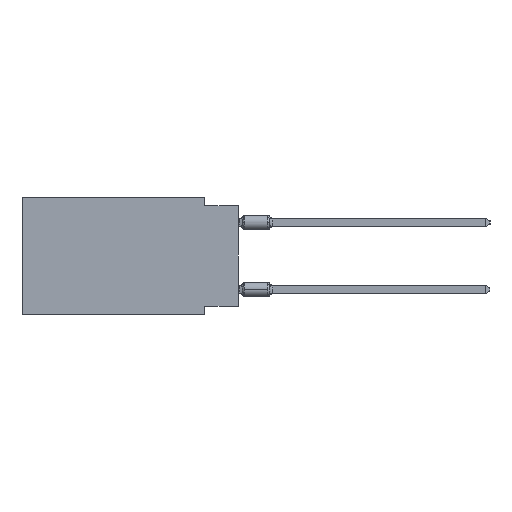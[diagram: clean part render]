
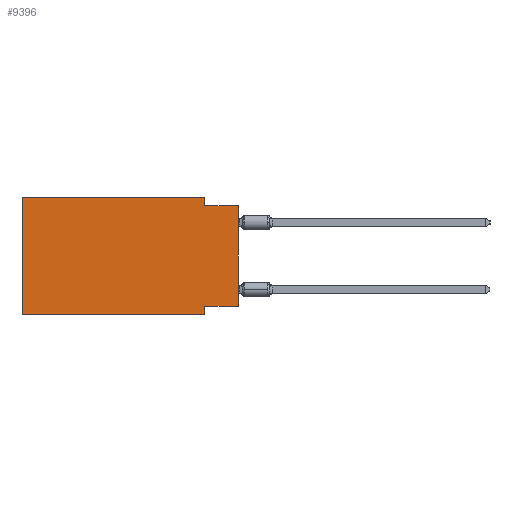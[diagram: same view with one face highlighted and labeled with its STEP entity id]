
A CAD part, left-side view. The second image highlights one B-rep face of the part: STEP entity #9396.
In plain terms, the highlighted planar face has unit normal (-1, 0, 0).
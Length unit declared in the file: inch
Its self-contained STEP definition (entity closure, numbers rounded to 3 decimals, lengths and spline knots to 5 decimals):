
#446 = CARTESIAN_POINT ( 'NONE',  ( 0., 0., -0.325 ) ) ;
#1252 = ORIENTED_EDGE ( 'NONE', *, *, #28286, .F. ) ;
#1313 = VECTOR ( 'NONE', #11956, 39.37008 ) ;
#2677 = CARTESIAN_POINT ( 'NONE',  ( 0., 0.1, -0.35 ) ) ;
#3009 = VERTEX_POINT ( 'NONE', #25775 ) ;
#3066 = DIRECTION ( 'NONE',  ( 0., 1., 0. ) ) ;
#3431 = DIRECTION ( 'NONE',  ( 0., -1., 0. ) ) ;
#3867 = EDGE_CURVE ( 'NONE', #3009, #34029, #23481, .T. ) ;
#5964 = AXIS2_PLACEMENT_3D ( 'NONE', #33407, #11883, #37676 ) ;
#6790 = VECTOR ( 'NONE', #33878, 39.37008 ) ;
#7600 = VERTEX_POINT ( 'NONE', #25044 ) ;
#8003 = VECTOR ( 'NONE', #27039, 39.37008 ) ;
#8285 = VERTEX_POINT ( 'NONE', #33639 ) ;
#9396 = ADVANCED_FACE ( 'NONE', ( #19673 ), #16127, .F. ) ;
#10119 = DIRECTION ( 'NONE',  ( 0., -1., 0. ) ) ;
#10926 = VERTEX_POINT ( 'NONE', #19369 ) ;
#11883 = DIRECTION ( 'NONE',  ( 1., 0., 0. ) ) ;
#11956 = DIRECTION ( 'NONE',  ( 0., 0., -1. ) ) ;
#13895 = CARTESIAN_POINT ( 'NONE',  ( 0., 0.645, -0.35 ) ) ;
#15711 = CARTESIAN_POINT ( 'NONE',  ( 0., 0.645, -0.35 ) ) ;
#16127 = PLANE ( 'NONE',  #5964 ) ;
#17143 = EDGE_CURVE ( 'NONE', #43151, #31957, #22496, .T. ) ;
#17479 = ORIENTED_EDGE ( 'NONE', *, *, #22959, .F. ) ;
#17889 = CARTESIAN_POINT ( 'NONE',  ( 0., 0.1, -0.025 ) ) ;
#18559 = CARTESIAN_POINT ( 'NONE',  ( 0., 0.645, 0. ) ) ;
#19369 = CARTESIAN_POINT ( 'NONE',  ( 0., 0.1, 0. ) ) ;
#19673 = FACE_OUTER_BOUND ( 'NONE', #28832, .T. ) ;
#20497 = VECTOR ( 'NONE', #3066, 39.37008 ) ;
#21859 = VECTOR ( 'NONE', #3431, 39.37008 ) ;
#21965 = LINE ( 'NONE', #446, #20497 ) ;
#22496 = LINE ( 'NONE', #37662, #6790 ) ;
#22507 = EDGE_CURVE ( 'NONE', #44842, #7600, #29139, .T. ) ;
#22959 = EDGE_CURVE ( 'NONE', #8285, #3009, #21965, .T. ) ;
#23430 = EDGE_CURVE ( 'NONE', #43151, #34029, #31881, .T. ) ;
#23481 = LINE ( 'NONE', #2677, #8003 ) ;
#24514 = LINE ( 'NONE', #42287, #38938 ) ;
#25044 = CARTESIAN_POINT ( 'NONE',  ( 0., 0., -0.025 ) ) ;
#25245 = ORIENTED_EDGE ( 'NONE', *, *, #17143, .F. ) ;
#25775 = CARTESIAN_POINT ( 'NONE',  ( 0., 0.1, -0.325 ) ) ;
#25798 = VECTOR ( 'NONE', #10119, 39.37008 ) ;
#27039 = DIRECTION ( 'NONE',  ( 0., 0., -1. ) ) ;
#27448 = ORIENTED_EDGE ( 'NONE', *, *, #37164, .F. ) ;
#27828 = ORIENTED_EDGE ( 'NONE', *, *, #23430, .T. ) ;
#28286 = EDGE_CURVE ( 'NONE', #10926, #44842, #40580, .T. ) ;
#28309 = ORIENTED_EDGE ( 'NONE', *, *, #43492, .T. ) ;
#28832 = EDGE_LOOP ( 'NONE', ( #28309, #33011, #1252, #27448, #25245, #27828, #40102, #17479 ) ) ;
#29139 = LINE ( 'NONE', #42876, #38626 ) ;
#29693 = CARTESIAN_POINT ( 'NONE',  ( 0., 0.1, 0. ) ) ;
#31881 = LINE ( 'NONE', #13895, #25798 ) ;
#31957 = VERTEX_POINT ( 'NONE', #44024 ) ;
#33011 = ORIENTED_EDGE ( 'NONE', *, *, #22507, .F. ) ;
#33178 = CARTESIAN_POINT ( 'NONE',  ( 0., 0.1, -0.35 ) ) ;
#33407 = CARTESIAN_POINT ( 'NONE',  ( 0., 0.645, 0. ) ) ;
#33639 = CARTESIAN_POINT ( 'NONE',  ( 0., 0., -0.325 ) ) ;
#33878 = DIRECTION ( 'NONE',  ( 0., 0., 1. ) ) ;
#34029 = VERTEX_POINT ( 'NONE', #33178 ) ;
#36321 = LINE ( 'NONE', #18559, #21859 ) ;
#37164 = EDGE_CURVE ( 'NONE', #31957, #10926, #36321, .T. ) ;
#37662 = CARTESIAN_POINT ( 'NONE',  ( 0., 0.645, 0. ) ) ;
#37676 = DIRECTION ( 'NONE',  ( 0., 0., -1. ) ) ;
#38266 = DIRECTION ( 'NONE',  ( 0., 0., 1. ) ) ;
#38626 = VECTOR ( 'NONE', #40021, 39.37008 ) ;
#38938 = VECTOR ( 'NONE', #38266, 39.37008 ) ;
#40021 = DIRECTION ( 'NONE',  ( 0., -1., 0. ) ) ;
#40102 = ORIENTED_EDGE ( 'NONE', *, *, #3867, .F. ) ;
#40580 = LINE ( 'NONE', #29693, #1313 ) ;
#42287 = CARTESIAN_POINT ( 'NONE',  ( 0., 0., 0. ) ) ;
#42876 = CARTESIAN_POINT ( 'NONE',  ( 0., 0., -0.025 ) ) ;
#43151 = VERTEX_POINT ( 'NONE', #15711 ) ;
#43492 = EDGE_CURVE ( 'NONE', #8285, #7600, #24514, .T. ) ;
#44024 = CARTESIAN_POINT ( 'NONE',  ( 0., 0.645, 0. ) ) ;
#44842 = VERTEX_POINT ( 'NONE', #17889 ) ;
